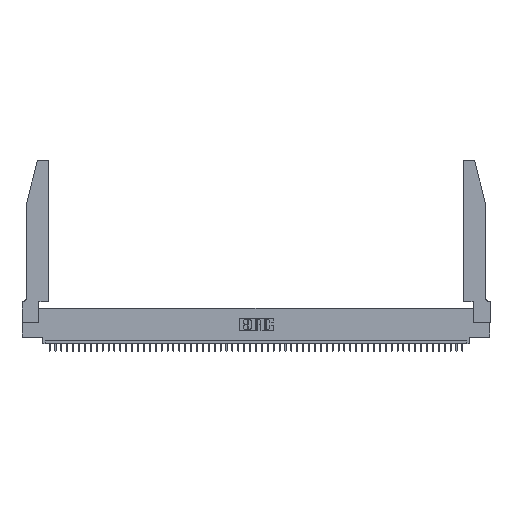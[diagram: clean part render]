
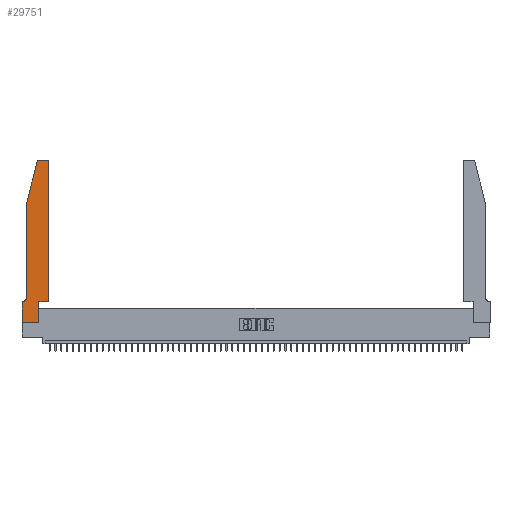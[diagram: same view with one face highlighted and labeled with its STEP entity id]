
A CAD part, top view. The second image highlights one B-rep face of the part: STEP entity #29751.
In plain terms, the highlighted planar face has unit normal (0, 0, 1).
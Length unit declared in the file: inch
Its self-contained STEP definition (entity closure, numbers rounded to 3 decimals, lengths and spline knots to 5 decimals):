
#73 = VERTEX_POINT ( 'NONE', #204 ) ;
#204 = CARTESIAN_POINT ( 'NONE',  ( 0.25487, 2.72718, 0.37 ) ) ;
#574 = DIRECTION ( 'NONE',  ( 0., 1., 0. ) ) ;
#1072 = EDGE_CURVE ( 'NONE', #45685, #25286, #46379, .T. ) ;
#1310 = DIRECTION ( 'NONE',  ( 1., 0., 0. ) ) ;
#1712 = VERTEX_POINT ( 'NONE', #16033 ) ;
#2583 = VECTOR ( 'NONE', #5359, 39.37008 ) ;
#3643 = ORIENTED_EDGE ( 'NONE', *, *, #18648, .T. ) ;
#4447 = EDGE_CURVE ( 'NONE', #38233, #46887, #38797, .T. ) ;
#4875 = EDGE_CURVE ( 'NONE', #25286, #1712, #45279, .T. ) ;
#5241 = VECTOR ( 'NONE', #26627, 39.37008 ) ;
#5359 = DIRECTION ( 'NONE',  ( 0., -1., 0. ) ) ;
#5935 = CARTESIAN_POINT ( 'NONE',  ( 0.2605, 2.75, 0.37 ) ) ;
#6051 = DIRECTION ( 'NONE',  ( 1., 0., 0. ) ) ;
#6273 = ORIENTED_EDGE ( 'NONE', *, *, #34907, .T. ) ;
#6488 = EDGE_CURVE ( 'NONE', #46887, #41908, #33866, .T. ) ;
#6695 = CARTESIAN_POINT ( 'NONE',  ( 0.284, 2.72, 0.37 ) ) ;
#7530 = CARTESIAN_POINT ( 'NONE',  ( 0., 0., 0.37 ) ) ;
#7545 = VERTEX_POINT ( 'NONE', #36162 ) ;
#8030 = CIRCLE ( 'NONE', #33539, 0.03 ) ;
#8327 = EDGE_CURVE ( 'NONE', #9012, #24659, #22492, .T. ) ;
#8844 = CARTESIAN_POINT ( 'NONE',  ( 0.4205, 2.75, 0.37 ) ) ;
#9012 = VERTEX_POINT ( 'NONE', #8844 ) ;
#10154 = CARTESIAN_POINT ( 'NONE',  ( 0., 0.35, 0.37 ) ) ;
#12056 = CARTESIAN_POINT ( 'NONE',  ( 0., 0., 0.37 ) ) ;
#12671 = CARTESIAN_POINT ( 'NONE',  ( 0., 0.35, 0.37 ) ) ;
#14198 = LINE ( 'NONE', #43135, #2583 ) ;
#14320 = VERTEX_POINT ( 'NONE', #38088 ) ;
#14511 = AXIS2_PLACEMENT_3D ( 'NONE', #6695, #23792, #35937 ) ;
#16033 = CARTESIAN_POINT ( 'NONE',  ( 0.2865, 0.35, 0.37 ) ) ;
#16521 = PLANE ( 'NONE',  #49929 ) ;
#18648 = EDGE_CURVE ( 'NONE', #41908, #45685, #40456, .T. ) ;
#19247 = ORIENTED_EDGE ( 'NONE', *, *, #6488, .T. ) ;
#19500 = DIRECTION ( 'NONE',  ( -0.239, -0.971, 0. ) ) ;
#20650 = VECTOR ( 'NONE', #1310, 39.37008 ) ;
#20991 = LINE ( 'NONE', #21268, #36703 ) ;
#21268 = CARTESIAN_POINT ( 'NONE',  ( 0.4505, 0.35, 0.37 ) ) ;
#22452 = ORIENTED_EDGE ( 'NONE', *, *, #52781, .T. ) ;
#22492 = LINE ( 'NONE', #5935, #5241 ) ;
#23792 = DIRECTION ( 'NONE',  ( 0., 0., 1. ) ) ;
#23849 = ORIENTED_EDGE ( 'NONE', *, *, #29415, .T. ) ;
#24171 = CIRCLE ( 'NONE', #14511, 0.03 ) ;
#24659 = VERTEX_POINT ( 'NONE', #52001 ) ;
#24778 = DIRECTION ( 'NONE',  ( 1., 0., 0. ) ) ;
#25286 = VERTEX_POINT ( 'NONE', #51013 ) ;
#25414 = CARTESIAN_POINT ( 'NONE',  ( 0., 0., 0.37 ) ) ;
#26627 = DIRECTION ( 'NONE',  ( -1., 0., 0. ) ) ;
#29050 = DIRECTION ( 'NONE',  ( 0., 0., -1. ) ) ;
#29144 = VECTOR ( 'NONE', #45008, 39.37008 ) ;
#29415 = EDGE_CURVE ( 'NONE', #30678, #14320, #20991, .T. ) ;
#29707 = CARTESIAN_POINT ( 'NONE',  ( 0.0755, 0.35, 0.37 ) ) ;
#29751 = ADVANCED_FACE ( 'NONE', ( #33603 ), #16521, .T. ) ;
#30678 = VERTEX_POINT ( 'NONE', #46979 ) ;
#31145 = CARTESIAN_POINT ( 'NONE',  ( 0.4205, 2.72, 0.37 ) ) ;
#31621 = VECTOR ( 'NONE', #19500, 39.37008 ) ;
#32102 = ORIENTED_EDGE ( 'NONE', *, *, #1072, .T. ) ;
#33539 = AXIS2_PLACEMENT_3D ( 'NONE', #31145, #47990, #6051 ) ;
#33603 = FACE_OUTER_BOUND ( 'NONE', #51237, .T. ) ;
#33866 = LINE ( 'NONE', #29707, #53505 ) ;
#34029 = ORIENTED_EDGE ( 'NONE', *, *, #40319, .T. ) ;
#34228 = DIRECTION ( 'NONE',  ( 1., 0., 0. ) ) ;
#34907 = EDGE_CURVE ( 'NONE', #1712, #30678, #47902, .T. ) ;
#35453 = EDGE_CURVE ( 'NONE', #24659, #73, #24171, .T. ) ;
#35937 = DIRECTION ( 'NONE',  ( 1., 0., 0. ) ) ;
#36162 = CARTESIAN_POINT ( 'NONE',  ( 0.0755, 2., 0.37 ) ) ;
#36703 = VECTOR ( 'NONE', #574, 39.37008 ) ;
#36839 = ORIENTED_EDGE ( 'NONE', *, *, #35453, .T. ) ;
#37142 = DIRECTION ( 'NONE',  ( 0., -1., 0. ) ) ;
#37789 = ORIENTED_EDGE ( 'NONE', *, *, #4447, .T. ) ;
#38088 = CARTESIAN_POINT ( 'NONE',  ( 0.4505, 2.72, 0.37 ) ) ;
#38233 = VERTEX_POINT ( 'NONE', #51268 ) ;
#38797 = CIRCLE ( 'NONE', #53792, 0.07 ) ;
#40319 = EDGE_CURVE ( 'NONE', #7545, #38233, #14198, .T. ) ;
#40452 = LINE ( 'NONE', #40719, #31621 ) ;
#40456 = LINE ( 'NONE', #12056, #46254 ) ;
#40719 = CARTESIAN_POINT ( 'NONE',  ( 0.0755, 2., 0.37 ) ) ;
#41467 = CARTESIAN_POINT ( 'NONE',  ( 0.0055, 0.42, 0.37 ) ) ;
#41776 = VECTOR ( 'NONE', #34228, 39.37008 ) ;
#41908 = VERTEX_POINT ( 'NONE', #10154 ) ;
#41982 = EDGE_CURVE ( 'NONE', #73, #7545, #40452, .T. ) ;
#43135 = CARTESIAN_POINT ( 'NONE',  ( 0.0755, 2., 0.37 ) ) ;
#45008 = DIRECTION ( 'NONE',  ( 0., 1., 0. ) ) ;
#45279 = LINE ( 'NONE', #49956, #29144 ) ;
#45609 = DIRECTION ( 'NONE',  ( -1., 0., 0. ) ) ;
#45685 = VERTEX_POINT ( 'NONE', #7530 ) ;
#46254 = VECTOR ( 'NONE', #37142, 39.37008 ) ;
#46379 = LINE ( 'NONE', #25414, #41776 ) ;
#46887 = VERTEX_POINT ( 'NONE', #49258 ) ;
#46979 = CARTESIAN_POINT ( 'NONE',  ( 0.4505, 0.35, 0.37 ) ) ;
#47355 = CARTESIAN_POINT ( 'NONE',  ( 0.4505, 0.35, 0.37 ) ) ;
#47902 = LINE ( 'NONE', #47355, #20650 ) ;
#47990 = DIRECTION ( 'NONE',  ( 0., 0., 1. ) ) ;
#49258 = CARTESIAN_POINT ( 'NONE',  ( 0.0055, 0.35, 0.37 ) ) ;
#49929 = AXIS2_PLACEMENT_3D ( 'NONE', #12671, #50437, #24778 ) ;
#49956 = CARTESIAN_POINT ( 'NONE',  ( 0.2865, 0.35, 0.37 ) ) ;
#50413 = ORIENTED_EDGE ( 'NONE', *, *, #4875, .T. ) ;
#50437 = DIRECTION ( 'NONE',  ( 0., 0., 1. ) ) ;
#51013 = CARTESIAN_POINT ( 'NONE',  ( 0.2865, 0., 0.37 ) ) ;
#51237 = EDGE_LOOP ( 'NONE', ( #54349, #36839, #51901, #34029, #37789, #19247, #3643, #32102, #50413, #6273, #23849, #22452 ) ) ;
#51268 = CARTESIAN_POINT ( 'NONE',  ( 0.0755, 0.42, 0.37 ) ) ;
#51512 = DIRECTION ( 'NONE',  ( -1., 0., 0. ) ) ;
#51901 = ORIENTED_EDGE ( 'NONE', *, *, #41982, .T. ) ;
#52001 = CARTESIAN_POINT ( 'NONE',  ( 0.284, 2.75, 0.37 ) ) ;
#52781 = EDGE_CURVE ( 'NONE', #14320, #9012, #8030, .T. ) ;
#53505 = VECTOR ( 'NONE', #51512, 39.37008 ) ;
#53792 = AXIS2_PLACEMENT_3D ( 'NONE', #41467, #29050, #45609 ) ;
#54349 = ORIENTED_EDGE ( 'NONE', *, *, #8327, .T. ) ;
